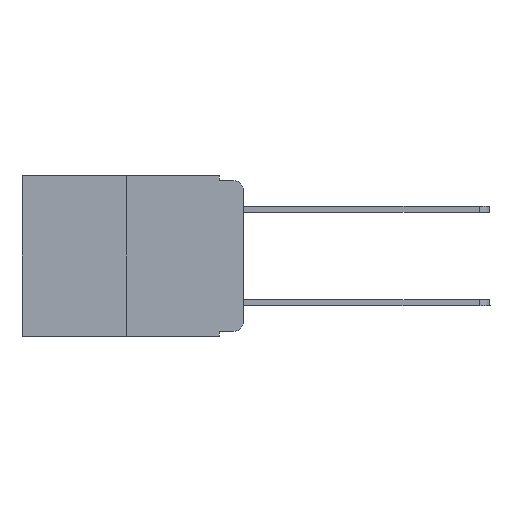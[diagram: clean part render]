
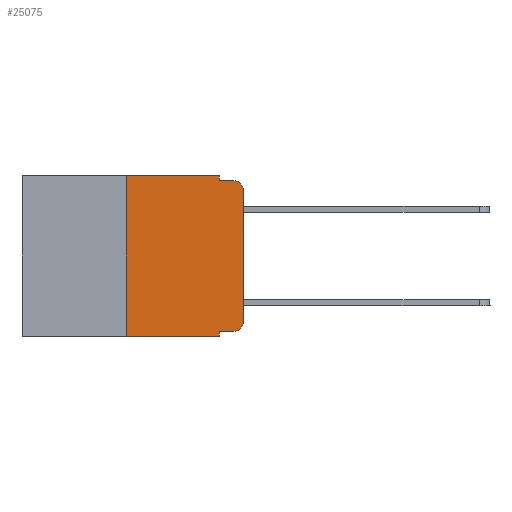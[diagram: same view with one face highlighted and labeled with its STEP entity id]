
A CAD part, left-side view. The second image highlights one B-rep face of the part: STEP entity #25075.
In plain terms, the highlighted planar face has unit normal (-1, 0, 0).
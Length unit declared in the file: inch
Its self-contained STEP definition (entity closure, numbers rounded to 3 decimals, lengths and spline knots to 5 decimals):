
#513 = EDGE_CURVE ( 'NONE', #22769, #20988, #19067, .T. ) ;
#535 = VERTEX_POINT ( 'NONE', #18542 ) ;
#1172 = LINE ( 'NONE', #25463, #25221 ) ;
#1304 = DIRECTION ( 'NONE',  ( -1., 0., 0. ) ) ;
#2536 = DIRECTION ( 'NONE',  ( 0., 0., 1. ) ) ;
#2894 = ORIENTED_EDGE ( 'NONE', *, *, #513, .F. ) ;
#3214 = DIRECTION ( 'NONE',  ( 0., -1., 0. ) ) ;
#3218 = CARTESIAN_POINT ( 'NONE',  ( 0., 0.473, 0. ) ) ;
#3875 = EDGE_CURVE ( 'NONE', #535, #24315, #8916, .T. ) ;
#4436 = LINE ( 'NONE', #15460, #14251 ) ;
#4569 = EDGE_CURVE ( 'NONE', #15605, #16134, #5755, .T. ) ;
#4752 = VECTOR ( 'NONE', #2536, 39.37008 ) ;
#4957 = PLANE ( 'NONE',  #10544 ) ;
#5370 = CIRCLE ( 'NONE', #13051, 0.02 ) ;
#5755 = LINE ( 'NONE', #10307, #20091 ) ;
#5814 = LINE ( 'NONE', #13947, #25341 ) ;
#5822 = EDGE_CURVE ( 'NONE', #19301, #16134, #1172, .T. ) ;
#6204 = CARTESIAN_POINT ( 'NONE',  ( 0., 0.25, -0.343 ) ) ;
#7446 = DIRECTION ( 'NONE',  ( 0., -1., 0. ) ) ;
#7991 = EDGE_CURVE ( 'NONE', #10154, #24315, #4436, .T. ) ;
#8204 = EDGE_LOOP ( 'NONE', ( #25004, #26255, #11168, #9233, #2894, #10619, #19956, #17865, #19805, #23731 ) ) ;
#8494 = DIRECTION ( 'NONE',  ( 0., -1., 0. ) ) ;
#8916 = CIRCLE ( 'NONE', #16125, 0.02 ) ;
#9233 = ORIENTED_EDGE ( 'NONE', *, *, #12545, .F. ) ;
#9406 = DIRECTION ( 'NONE',  ( 0., -1., 0. ) ) ;
#9407 = CARTESIAN_POINT ( 'NONE',  ( 0., 0.02, -0.03 ) ) ;
#9546 = DIRECTION ( 'NONE',  ( 0., 0., -1. ) ) ;
#10154 = VERTEX_POINT ( 'NONE', #21547 ) ;
#10218 = CARTESIAN_POINT ( 'NONE',  ( 0., 0.02, -0.01 ) ) ;
#10307 = CARTESIAN_POINT ( 'NONE',  ( 0., 0.051, 0. ) ) ;
#10544 = AXIS2_PLACEMENT_3D ( 'NONE', #3218, #13473, #21159 ) ;
#10619 = ORIENTED_EDGE ( 'NONE', *, *, #19129, .F. ) ;
#10684 = VERTEX_POINT ( 'NONE', #13716 ) ;
#11168 = ORIENTED_EDGE ( 'NONE', *, *, #7991, .F. ) ;
#12483 = CARTESIAN_POINT ( 'NONE',  ( 0., 0.473, 0. ) ) ;
#12545 = EDGE_CURVE ( 'NONE', #20988, #10154, #5814, .T. ) ;
#13051 = AXIS2_PLACEMENT_3D ( 'NONE', #19226, #15663, #9546 ) ;
#13402 = CARTESIAN_POINT ( 'NONE',  ( 0., 0.051, -0.333 ) ) ;
#13473 = DIRECTION ( 'NONE',  ( 1., 0., 0. ) ) ;
#13716 = CARTESIAN_POINT ( 'NONE',  ( 0., 0., -0.313 ) ) ;
#13745 = VECTOR ( 'NONE', #8494, 39.37008 ) ;
#13922 = CARTESIAN_POINT ( 'NONE',  ( 0., 0.051, 0. ) ) ;
#13947 = CARTESIAN_POINT ( 'NONE',  ( 0., 0.051, 0. ) ) ;
#14251 = VECTOR ( 'NONE', #3214, 39.37008 ) ;
#14328 = VERTEX_POINT ( 'NONE', #20962 ) ;
#15011 = CARTESIAN_POINT ( 'NONE',  ( 0., 0.25, 0. ) ) ;
#15038 = LINE ( 'NONE', #23128, #19168 ) ;
#15460 = CARTESIAN_POINT ( 'NONE',  ( 0., 0.051, -0.01 ) ) ;
#15605 = VERTEX_POINT ( 'NONE', #13402 ) ;
#15663 = DIRECTION ( 'NONE',  ( -1., 0., 0. ) ) ;
#15947 = DIRECTION ( 'NONE',  ( 0., 0., -1. ) ) ;
#16125 = AXIS2_PLACEMENT_3D ( 'NONE', #9407, #1304, #24005 ) ;
#16134 = VERTEX_POINT ( 'NONE', #21189 ) ;
#16372 = LINE ( 'NONE', #20608, #4752 ) ;
#17132 = EDGE_CURVE ( 'NONE', #15605, #14328, #25629, .T. ) ;
#17865 = ORIENTED_EDGE ( 'NONE', *, *, #4569, .F. ) ;
#18542 = CARTESIAN_POINT ( 'NONE',  ( 0., 0., -0.03 ) ) ;
#19067 = LINE ( 'NONE', #12483, #13745 ) ;
#19129 = EDGE_CURVE ( 'NONE', #19301, #22769, #15038, .T. ) ;
#19168 = VECTOR ( 'NONE', #19374, 39.37008 ) ;
#19226 = CARTESIAN_POINT ( 'NONE',  ( 0., 0.02, -0.313 ) ) ;
#19289 = FACE_OUTER_BOUND ( 'NONE', #8204, .T. ) ;
#19301 = VERTEX_POINT ( 'NONE', #6204 ) ;
#19374 = DIRECTION ( 'NONE',  ( 0., 0., 1. ) ) ;
#19805 = ORIENTED_EDGE ( 'NONE', *, *, #17132, .T. ) ;
#19956 = ORIENTED_EDGE ( 'NONE', *, *, #5822, .T. ) ;
#20091 = VECTOR ( 'NONE', #26086, 39.37008 ) ;
#20187 = EDGE_CURVE ( 'NONE', #10684, #535, #16372, .T. ) ;
#20608 = CARTESIAN_POINT ( 'NONE',  ( 0., 0., 0. ) ) ;
#20962 = CARTESIAN_POINT ( 'NONE',  ( 0., 0.02, -0.333 ) ) ;
#20988 = VERTEX_POINT ( 'NONE', #13922 ) ;
#21159 = DIRECTION ( 'NONE',  ( 0., 0., -1. ) ) ;
#21189 = CARTESIAN_POINT ( 'NONE',  ( 0., 0.051, -0.343 ) ) ;
#21547 = CARTESIAN_POINT ( 'NONE',  ( 0., 0.051, -0.01 ) ) ;
#22769 = VERTEX_POINT ( 'NONE', #15011 ) ;
#22936 = VECTOR ( 'NONE', #7446, 39.37008 ) ;
#23128 = CARTESIAN_POINT ( 'NONE',  ( 0., 0.25, 0. ) ) ;
#23731 = ORIENTED_EDGE ( 'NONE', *, *, #24245, .T. ) ;
#23786 = CARTESIAN_POINT ( 'NONE',  ( 0., 0.051, -0.333 ) ) ;
#24005 = DIRECTION ( 'NONE',  ( 0., 0., -1. ) ) ;
#24245 = EDGE_CURVE ( 'NONE', #14328, #10684, #5370, .T. ) ;
#24315 = VERTEX_POINT ( 'NONE', #10218 ) ;
#25004 = ORIENTED_EDGE ( 'NONE', *, *, #20187, .T. ) ;
#25075 = ADVANCED_FACE ( 'NONE', ( #19289 ), #4957, .F. ) ;
#25221 = VECTOR ( 'NONE', #9406, 39.37008 ) ;
#25341 = VECTOR ( 'NONE', #15947, 39.37008 ) ;
#25463 = CARTESIAN_POINT ( 'NONE',  ( 0., 0.473, -0.343 ) ) ;
#25629 = LINE ( 'NONE', #23786, #22936 ) ;
#26086 = DIRECTION ( 'NONE',  ( 0., 0., -1. ) ) ;
#26255 = ORIENTED_EDGE ( 'NONE', *, *, #3875, .T. ) ;
